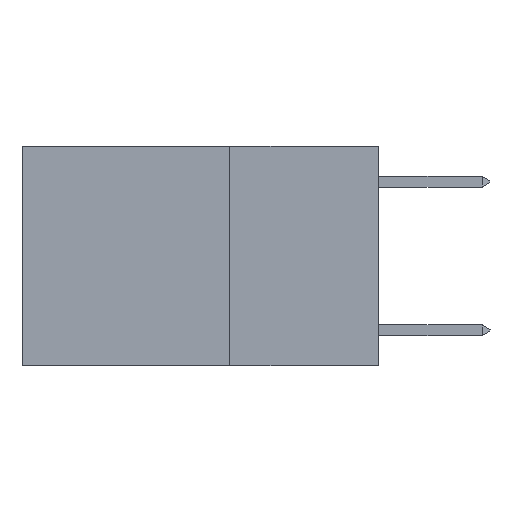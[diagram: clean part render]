
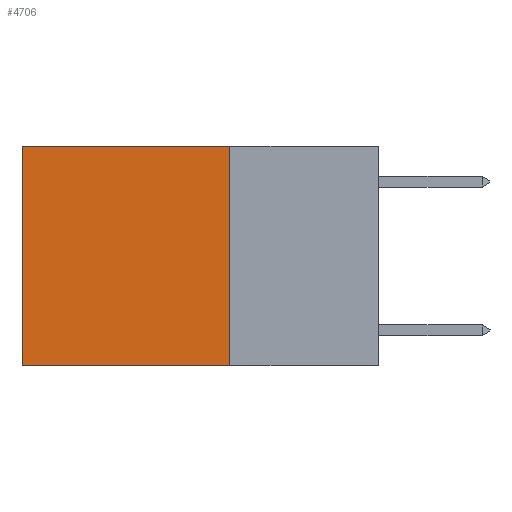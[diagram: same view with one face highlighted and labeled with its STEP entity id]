
A CAD part, left-side view. The second image highlights one B-rep face of the part: STEP entity #4706.
In plain terms, the highlighted planar face has unit normal (-1, 0, 0).
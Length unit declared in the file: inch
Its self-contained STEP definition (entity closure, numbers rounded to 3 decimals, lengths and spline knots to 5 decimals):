
#271 = VERTEX_POINT ( 'NONE', #1992 ) ;
#624 = ORIENTED_EDGE ( 'NONE', *, *, #25629, .F. ) ;
#1151 = EDGE_CURVE ( 'NONE', #4086, #5232, #19591, .T. ) ;
#1276 = EDGE_CURVE ( 'NONE', #9171, #271, #18981, .T. ) ;
#1992 = CARTESIAN_POINT ( 'NONE',  ( 0.2625, 0.6, -0.37 ) ) ;
#4086 = VERTEX_POINT ( 'NONE', #19835 ) ;
#4262 = LINE ( 'NONE', #23253, #4767 ) ;
#4706 = ADVANCED_FACE ( 'NONE', ( #20060 ), #19413, .F. ) ;
#4767 = VECTOR ( 'NONE', #22999, 39.37008 ) ;
#5232 = VERTEX_POINT ( 'NONE', #7089 ) ;
#5399 = ORIENTED_EDGE ( 'NONE', *, *, #9894, .T. ) ;
#6330 = AXIS2_PLACEMENT_3D ( 'NONE', #19672, #19231, #19149 ) ;
#6985 = CARTESIAN_POINT ( 'NONE',  ( 0.2625, 0.6, 0. ) ) ;
#7089 = CARTESIAN_POINT ( 'NONE',  ( 0.2625, 0.25, -0.37 ) ) ;
#7269 = EDGE_LOOP ( 'NONE', ( #17003, #624, #9437, #5399 ) ) ;
#8478 = CARTESIAN_POINT ( 'NONE',  ( 0.2625, 0.6, 0. ) ) ;
#9171 = VERTEX_POINT ( 'NONE', #6985 ) ;
#9425 = DIRECTION ( 'NONE',  ( 0., 0., -1. ) ) ;
#9437 = ORIENTED_EDGE ( 'NONE', *, *, #1151, .F. ) ;
#9894 = EDGE_CURVE ( 'NONE', #4086, #9171, #4262, .T. ) ;
#15821 = DIRECTION ( 'NONE',  ( 0., 1., 0. ) ) ;
#16079 = VECTOR ( 'NONE', #15821, 39.37008 ) ;
#16389 = LINE ( 'NONE', #17792, #16079 ) ;
#17003 = ORIENTED_EDGE ( 'NONE', *, *, #1276, .T. ) ;
#17748 = DIRECTION ( 'NONE',  ( 0., 0., -1. ) ) ;
#17792 = CARTESIAN_POINT ( 'NONE',  ( 0.2625, 0.25, -0.37 ) ) ;
#18954 = VECTOR ( 'NONE', #9425, 39.37008 ) ;
#18981 = LINE ( 'NONE', #8478, #18954 ) ;
#19149 = DIRECTION ( 'NONE',  ( 0., 0., -1. ) ) ;
#19231 = DIRECTION ( 'NONE',  ( 1., 0., 0. ) ) ;
#19413 = PLANE ( 'NONE',  #6330 ) ;
#19543 = VECTOR ( 'NONE', #17748, 39.37008 ) ;
#19591 = LINE ( 'NONE', #19629, #19543 ) ;
#19629 = CARTESIAN_POINT ( 'NONE',  ( 0.2625, 0.25, 0. ) ) ;
#19672 = CARTESIAN_POINT ( 'NONE',  ( 0.2625, 0.25, 0. ) ) ;
#19835 = CARTESIAN_POINT ( 'NONE',  ( 0.2625, 0.25, 0. ) ) ;
#20060 = FACE_OUTER_BOUND ( 'NONE', #7269, .T. ) ;
#22999 = DIRECTION ( 'NONE',  ( 0., 1., 0. ) ) ;
#23253 = CARTESIAN_POINT ( 'NONE',  ( 0.2625, 0.25, 0. ) ) ;
#25629 = EDGE_CURVE ( 'NONE', #5232, #271, #16389, .T. ) ;
